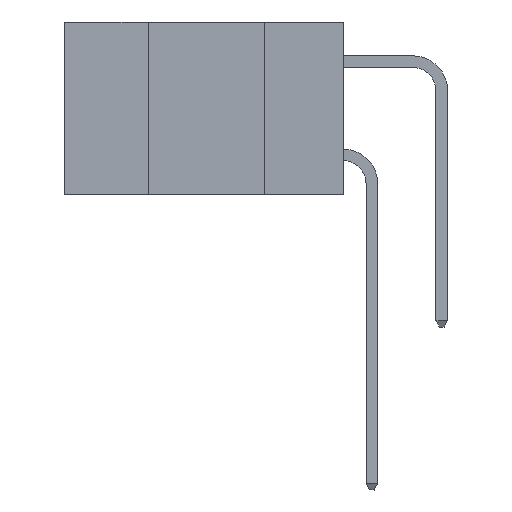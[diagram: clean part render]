
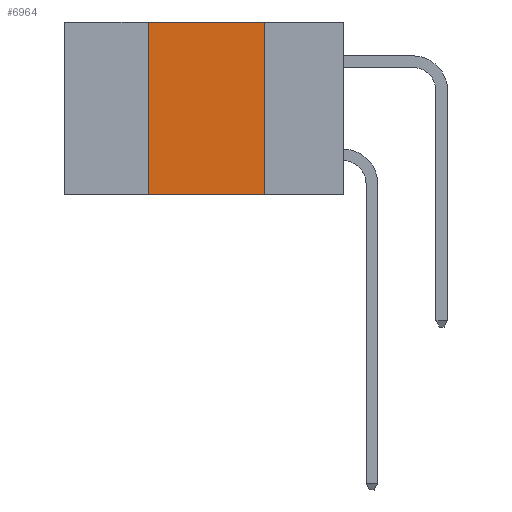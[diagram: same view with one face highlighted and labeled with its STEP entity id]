
A CAD part, left-side view. The second image highlights one B-rep face of the part: STEP entity #6964.
In plain terms, the highlighted planar face has unit normal (-1, 0, 0).
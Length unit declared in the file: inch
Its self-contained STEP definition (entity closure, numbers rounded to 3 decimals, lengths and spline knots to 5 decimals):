
#274 = ORIENTED_EDGE ( 'NONE', *, *, #1404, .F. ) ;
#398 = DIRECTION ( 'NONE',  ( 0., -1., 0. ) ) ;
#928 = DIRECTION ( 'NONE',  ( 1., 0., 0. ) ) ;
#1138 = VECTOR ( 'NONE', #11789, 39.37008 ) ;
#1230 = CARTESIAN_POINT ( 'NONE',  ( 0., 0.42, 0. ) ) ;
#1404 = EDGE_CURVE ( 'NONE', #10467, #10930, #9045, .T. ) ;
#2087 = CARTESIAN_POINT ( 'NONE',  ( 0., 0.17, -0.37 ) ) ;
#2678 = FACE_OUTER_BOUND ( 'NONE', #4981, .T. ) ;
#2679 = VECTOR ( 'NONE', #6320, 39.37008 ) ;
#3126 = LINE ( 'NONE', #8037, #1138 ) ;
#3162 = LINE ( 'NONE', #3404, #5106 ) ;
#3404 = CARTESIAN_POINT ( 'NONE',  ( 0., 0.42, -0.37 ) ) ;
#3541 = CARTESIAN_POINT ( 'NONE',  ( 0., 0.17, -0.37 ) ) ;
#3726 = ORIENTED_EDGE ( 'NONE', *, *, #10487, .F. ) ;
#4981 = EDGE_LOOP ( 'NONE', ( #6398, #274, #3726, #10651 ) ) ;
#5106 = VECTOR ( 'NONE', #10713, 39.37008 ) ;
#5630 = CARTESIAN_POINT ( 'NONE',  ( 0., 0.6, 0. ) ) ;
#6033 = CARTESIAN_POINT ( 'NONE',  ( 0., 0.6, 0. ) ) ;
#6084 = LINE ( 'NONE', #3541, #2679 ) ;
#6320 = DIRECTION ( 'NONE',  ( 0., 0., -1. ) ) ;
#6387 = VERTEX_POINT ( 'NONE', #10839 ) ;
#6398 = ORIENTED_EDGE ( 'NONE', *, *, #6856, .F. ) ;
#6856 = EDGE_CURVE ( 'NONE', #10930, #8082, #6084, .T. ) ;
#6964 = ADVANCED_FACE ( 'NONE', ( #2678 ), #8392, .F. ) ;
#7552 = DIRECTION ( 'NONE',  ( 0., 0., -1. ) ) ;
#8037 = CARTESIAN_POINT ( 'NONE',  ( 0., 0.6, -0.37 ) ) ;
#8082 = VERTEX_POINT ( 'NONE', #2087 ) ;
#8174 = AXIS2_PLACEMENT_3D ( 'NONE', #5630, #928, #7552 ) ;
#8319 = VECTOR ( 'NONE', #398, 39.37008 ) ;
#8392 = PLANE ( 'NONE',  #8174 ) ;
#8806 = CARTESIAN_POINT ( 'NONE',  ( 0., 0.17, 0. ) ) ;
#9045 = LINE ( 'NONE', #6033, #8319 ) ;
#10467 = VERTEX_POINT ( 'NONE', #1230 ) ;
#10487 = EDGE_CURVE ( 'NONE', #6387, #10467, #3162, .T. ) ;
#10651 = ORIENTED_EDGE ( 'NONE', *, *, #11859, .T. ) ;
#10713 = DIRECTION ( 'NONE',  ( 0., 0., 1. ) ) ;
#10839 = CARTESIAN_POINT ( 'NONE',  ( 0., 0.42, -0.37 ) ) ;
#10930 = VERTEX_POINT ( 'NONE', #8806 ) ;
#11789 = DIRECTION ( 'NONE',  ( 0., -1., 0. ) ) ;
#11859 = EDGE_CURVE ( 'NONE', #6387, #8082, #3126, .T. ) ;
